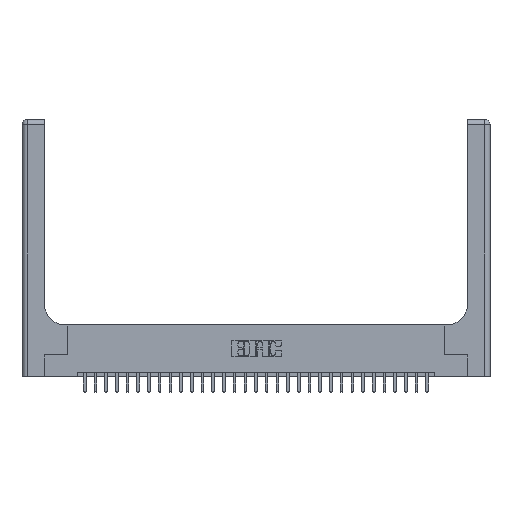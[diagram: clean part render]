
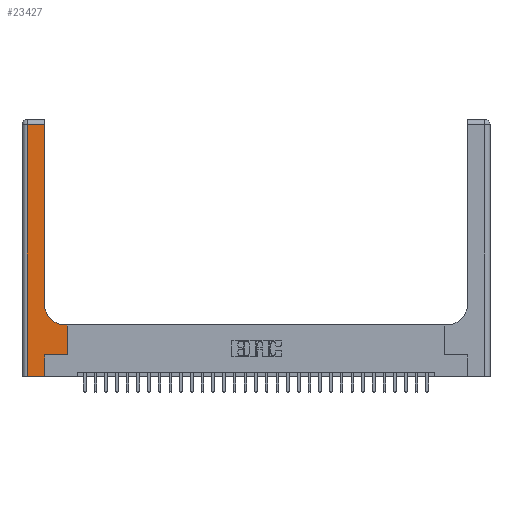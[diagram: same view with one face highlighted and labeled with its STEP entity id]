
A CAD part, top view. The second image highlights one B-rep face of the part: STEP entity #23427.
In plain terms, the highlighted planar face has unit normal (0, 0, 1).
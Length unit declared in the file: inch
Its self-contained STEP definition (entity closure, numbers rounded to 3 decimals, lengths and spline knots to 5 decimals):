
#148 = CARTESIAN_POINT ( 'NONE',  ( 0., 3., 0.37 ) ) ;
#287 = LINE ( 'NONE', #23371, #13269 ) ;
#838 = LINE ( 'NONE', #25736, #23869 ) ;
#1326 = ORIENTED_EDGE ( 'NONE', *, *, #8883, .T. ) ;
#2032 = ORIENTED_EDGE ( 'NONE', *, *, #24427, .T. ) ;
#2338 = DIRECTION ( 'NONE',  ( -1., 0., 0. ) ) ;
#3242 = LINE ( 'NONE', #19172, #15523 ) ;
#3373 = VERTEX_POINT ( 'NONE', #25551 ) ;
#3551 = EDGE_CURVE ( 'NONE', #20100, #16867, #25159, .T. ) ;
#3559 = AXIS2_PLACEMENT_3D ( 'NONE', #148, #19571, #2338 ) ;
#4148 = CARTESIAN_POINT ( 'NONE',  ( 0., 0., 0.37 ) ) ;
#5195 = LINE ( 'NONE', #13919, #8614 ) ;
#5308 = EDGE_CURVE ( 'NONE', #3373, #10534, #13717, .T. ) ;
#5403 = EDGE_CURVE ( 'NONE', #12778, #3373, #5570, .T. ) ;
#5570 = LINE ( 'NONE', #18235, #18800 ) ;
#5765 = VERTEX_POINT ( 'NONE', #22539 ) ;
#6219 = DIRECTION ( 'NONE',  ( 0., 1., 0. ) ) ;
#6401 = DIRECTION ( 'NONE',  ( 0., 0., -1. ) ) ;
#7270 = ORIENTED_EDGE ( 'NONE', *, *, #11160, .T. ) ;
#7443 = CARTESIAN_POINT ( 'NONE',  ( 0.265, 0.25, 0.37 ) ) ;
#8284 = DIRECTION ( 'NONE',  ( 0., -1., 0. ) ) ;
#8614 = VECTOR ( 'NONE', #20487, 39.37008 ) ;
#8883 = EDGE_CURVE ( 'NONE', #5765, #20100, #3242, .T. ) ;
#9030 = VECTOR ( 'NONE', #23786, 39.37008 ) ;
#9075 = CARTESIAN_POINT ( 'NONE',  ( 0.265, 0.25, 0.37 ) ) ;
#9168 = FACE_OUTER_BOUND ( 'NONE', #17772, .T. ) ;
#9673 = AXIS2_PLACEMENT_3D ( 'NONE', #13147, #6401, #19508 ) ;
#9984 = ORIENTED_EDGE ( 'NONE', *, *, #5403, .T. ) ;
#10534 = VERTEX_POINT ( 'NONE', #13923 ) ;
#11065 = VERTEX_POINT ( 'NONE', #9075 ) ;
#11160 = EDGE_CURVE ( 'NONE', #11065, #27220, #13459, .T. ) ;
#11322 = PLANE ( 'NONE',  #3559 ) ;
#11814 = VECTOR ( 'NONE', #6219, 39.37008 ) ;
#12683 = DIRECTION ( 'NONE',  ( 0., 1., 0. ) ) ;
#12778 = VERTEX_POINT ( 'NONE', #15527 ) ;
#13117 = EDGE_CURVE ( 'NONE', #10534, #11065, #16244, .T. ) ;
#13147 = CARTESIAN_POINT ( 'NONE',  ( 0.51, 0.85, 0.37 ) ) ;
#13269 = VECTOR ( 'NONE', #12683, 39.37008 ) ;
#13459 = LINE ( 'NONE', #7443, #9030 ) ;
#13717 = LINE ( 'NONE', #4148, #15786 ) ;
#13919 = CARTESIAN_POINT ( 'NONE',  ( 0., 2.94, 0.37 ) ) ;
#13923 = CARTESIAN_POINT ( 'NONE',  ( 0.265, 0., 0.37 ) ) ;
#14061 = EDGE_CURVE ( 'NONE', #19938, #12778, #5195, .T. ) ;
#14474 = DIRECTION ( 'NONE',  ( -1., 0., 0. ) ) ;
#14661 = ORIENTED_EDGE ( 'NONE', *, *, #5308, .T. ) ;
#15369 = ORIENTED_EDGE ( 'NONE', *, *, #3551, .T. ) ;
#15523 = VECTOR ( 'NONE', #14474, 39.37008 ) ;
#15527 = CARTESIAN_POINT ( 'NONE',  ( 0.06, 2.94, 0.37 ) ) ;
#15786 = VECTOR ( 'NONE', #28075, 39.37008 ) ;
#16244 = LINE ( 'NONE', #23281, #11814 ) ;
#16401 = ORIENTED_EDGE ( 'NONE', *, *, #13117, .T. ) ;
#16867 = VERTEX_POINT ( 'NONE', #27634 ) ;
#17025 = DIRECTION ( 'NONE',  ( 0., 1., 0. ) ) ;
#17598 = CARTESIAN_POINT ( 'NONE',  ( 0.528, 0.25, 0.37 ) ) ;
#17750 = ORIENTED_EDGE ( 'NONE', *, *, #26468, .T. ) ;
#17772 = EDGE_LOOP ( 'NONE', ( #17750, #19742, #9984, #14661, #16401, #7270, #2032, #1326, #15369 ) ) ;
#18235 = CARTESIAN_POINT ( 'NONE',  ( 0.06, 3., 0.37 ) ) ;
#18800 = VECTOR ( 'NONE', #8284, 39.37008 ) ;
#19172 = CARTESIAN_POINT ( 'NONE',  ( 0.26, 0.6, 0.37 ) ) ;
#19466 = CARTESIAN_POINT ( 'NONE',  ( 0.51, 0.6, 0.37 ) ) ;
#19508 = DIRECTION ( 'NONE',  ( 1., 0., 0. ) ) ;
#19571 = DIRECTION ( 'NONE',  ( 0., 0., -1. ) ) ;
#19742 = ORIENTED_EDGE ( 'NONE', *, *, #14061, .T. ) ;
#19938 = VERTEX_POINT ( 'NONE', #22557 ) ;
#20100 = VERTEX_POINT ( 'NONE', #19466 ) ;
#20487 = DIRECTION ( 'NONE',  ( -1., 0., 0. ) ) ;
#22539 = CARTESIAN_POINT ( 'NONE',  ( 0.528, 0.6, 0.37 ) ) ;
#22557 = CARTESIAN_POINT ( 'NONE',  ( 0.26, 2.94, 0.37 ) ) ;
#23281 = CARTESIAN_POINT ( 'NONE',  ( 0.265, 0., 0.37 ) ) ;
#23371 = CARTESIAN_POINT ( 'NONE',  ( 0.528, 0.25, 0.37 ) ) ;
#23427 = ADVANCED_FACE ( 'NONE', ( #9168 ), #11322, .F. ) ;
#23786 = DIRECTION ( 'NONE',  ( 1., 0., 0. ) ) ;
#23869 = VECTOR ( 'NONE', #17025, 39.37008 ) ;
#24427 = EDGE_CURVE ( 'NONE', #27220, #5765, #287, .T. ) ;
#25159 = CIRCLE ( 'NONE', #9673, 0.25 ) ;
#25551 = CARTESIAN_POINT ( 'NONE',  ( 0.06, 0., 0.37 ) ) ;
#25736 = CARTESIAN_POINT ( 'NONE',  ( 0.26, 3., 0.37 ) ) ;
#26468 = EDGE_CURVE ( 'NONE', #16867, #19938, #838, .T. ) ;
#27220 = VERTEX_POINT ( 'NONE', #17598 ) ;
#27634 = CARTESIAN_POINT ( 'NONE',  ( 0.26, 0.85, 0.37 ) ) ;
#28075 = DIRECTION ( 'NONE',  ( 1., 0., 0. ) ) ;
